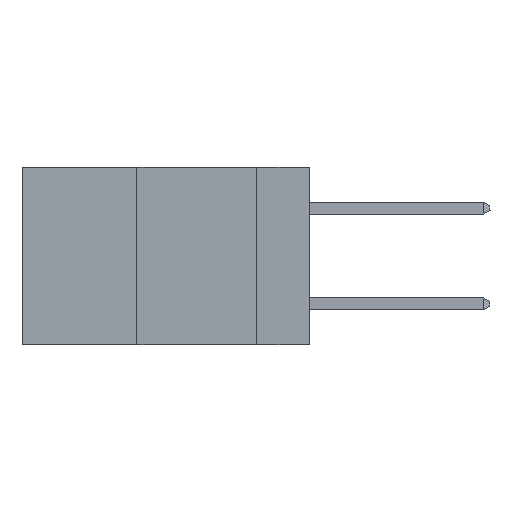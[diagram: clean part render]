
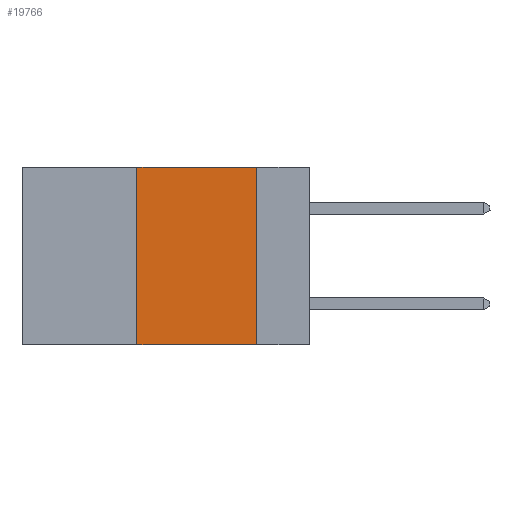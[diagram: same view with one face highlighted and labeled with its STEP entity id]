
A CAD part, left-side view. The second image highlights one B-rep face of the part: STEP entity #19766.
In plain terms, the highlighted planar face has unit normal (-1, 0, 0).
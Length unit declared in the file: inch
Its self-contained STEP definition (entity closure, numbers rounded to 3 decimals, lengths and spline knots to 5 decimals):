
#3883 = DIRECTION ( 'NONE',  ( 0., -1., 0. ) ) ;
#4039 = LINE ( 'NONE', #17017, #6900 ) ;
#4285 = DIRECTION ( 'NONE',  ( 0., 0., 1. ) ) ;
#4352 = DIRECTION ( 'NONE',  ( 0., 0., -1. ) ) ;
#4524 = ORIENTED_EDGE ( 'NONE', *, *, #19019, .F. ) ;
#4617 = AXIS2_PLACEMENT_3D ( 'NONE', #40282, #23691, #4352 ) ;
#5077 = ORIENTED_EDGE ( 'NONE', *, *, #11408, .F. ) ;
#6900 = VECTOR ( 'NONE', #36794, 39.37008 ) ;
#7972 = PLANE ( 'NONE',  #4617 ) ;
#8602 = CARTESIAN_POINT ( 'NONE',  ( 0., 0.11, -0.37 ) ) ;
#10549 = VECTOR ( 'NONE', #16671, 39.37008 ) ;
#11086 = CARTESIAN_POINT ( 'NONE',  ( 0., 0.36, 0. ) ) ;
#11408 = EDGE_CURVE ( 'NONE', #33926, #36293, #23006, .T. ) ;
#12007 = VECTOR ( 'NONE', #4285, 39.37008 ) ;
#12836 = LINE ( 'NONE', #29641, #10549 ) ;
#14143 = VERTEX_POINT ( 'NONE', #30053 ) ;
#16671 = DIRECTION ( 'NONE',  ( 0., -1., 0. ) ) ;
#17017 = CARTESIAN_POINT ( 'NONE',  ( 0., 0.11, 0. ) ) ;
#18025 = CARTESIAN_POINT ( 'NONE',  ( 0., 0.36, 0. ) ) ;
#18183 = VERTEX_POINT ( 'NONE', #8602 ) ;
#19019 = EDGE_CURVE ( 'NONE', #36293, #18183, #4039, .T. ) ;
#19766 = ADVANCED_FACE ( 'NONE', ( #27305 ), #7972, .F. ) ;
#23006 = LINE ( 'NONE', #30447, #30501 ) ;
#23691 = DIRECTION ( 'NONE',  ( 1., 0., 0. ) ) ;
#27305 = FACE_OUTER_BOUND ( 'NONE', #35397, .T. ) ;
#29641 = CARTESIAN_POINT ( 'NONE',  ( 0., 0.6, -0.37 ) ) ;
#30053 = CARTESIAN_POINT ( 'NONE',  ( 0., 0.36, -0.37 ) ) ;
#30447 = CARTESIAN_POINT ( 'NONE',  ( 0., 0.6, 0. ) ) ;
#30501 = VECTOR ( 'NONE', #3883, 39.37008 ) ;
#30979 = EDGE_CURVE ( 'NONE', #14143, #18183, #12836, .T. ) ;
#33191 = LINE ( 'NONE', #11086, #12007 ) ;
#33412 = EDGE_CURVE ( 'NONE', #14143, #33926, #33191, .T. ) ;
#33467 = ORIENTED_EDGE ( 'NONE', *, *, #33412, .F. ) ;
#33926 = VERTEX_POINT ( 'NONE', #18025 ) ;
#34393 = ORIENTED_EDGE ( 'NONE', *, *, #30979, .T. ) ;
#35397 = EDGE_LOOP ( 'NONE', ( #4524, #5077, #33467, #34393 ) ) ;
#36293 = VERTEX_POINT ( 'NONE', #37277 ) ;
#36794 = DIRECTION ( 'NONE',  ( 0., 0., -1. ) ) ;
#37277 = CARTESIAN_POINT ( 'NONE',  ( 0., 0.11, 0. ) ) ;
#40282 = CARTESIAN_POINT ( 'NONE',  ( 0., 0.6, 0. ) ) ;
